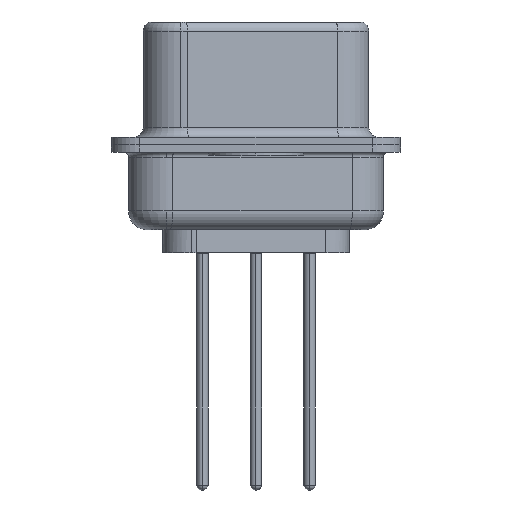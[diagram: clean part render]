
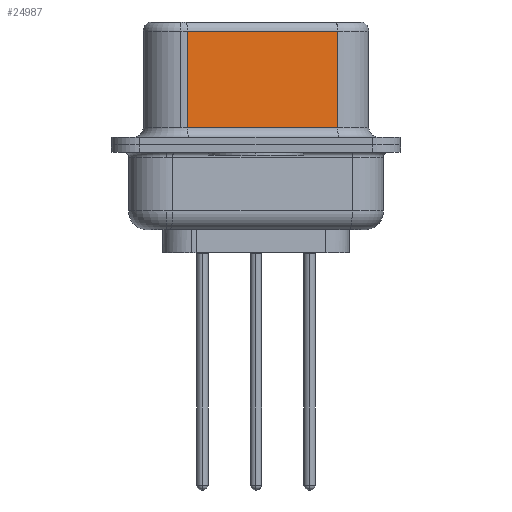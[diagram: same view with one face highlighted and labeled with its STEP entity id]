
A CAD part, left-side view. The second image highlights one B-rep face of the part: STEP entity #24987.
In plain terms, the highlighted planar face has unit normal (-0.985, -0.174, 0).
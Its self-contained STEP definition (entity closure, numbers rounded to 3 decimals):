
#434 = CARTESIAN_POINT ( 'NONE',  ( 5.132, -4.322, 0.9 ) ) ;
#1413 = ORIENTED_EDGE ( 'NONE', *, *, #6745, .T. ) ;
#2491 = VECTOR ( 'NONE', #8895, 1000. ) ;
#4350 = EDGE_CURVE ( 'NONE', #9837, #22912, #19893, .T. ) ;
#5107 = DIRECTION ( 'NONE',  ( 0., 0., -1. ) ) ;
#5774 = DIRECTION ( 'NONE',  ( 0.985, 0.174, 0. ) ) ;
#5904 = CARTESIAN_POINT ( 'NONE',  ( 5.132, -4.322, 6.52 ) ) ;
#6505 = VERTEX_POINT ( 'NONE', #16084 ) ;
#6745 = EDGE_CURVE ( 'NONE', #22912, #12935, #11440, .T. ) ;
#8169 = EDGE_CURVE ( 'NONE', #12935, #6505, #19488, .T. ) ;
#8642 = CARTESIAN_POINT ( 'NONE',  ( 3.73, 3.628, 0.9 ) ) ;
#8895 = DIRECTION ( 'NONE',  ( 0.174, -0.985, 0. ) ) ;
#9201 = CARTESIAN_POINT ( 'NONE',  ( 3.73, 3.628, 6.52 ) ) ;
#9265 = EDGE_LOOP ( 'NONE', ( #17857, #27466, #1413, #10239 ) ) ;
#9506 = VECTOR ( 'NONE', #10115, 1000. ) ;
#9744 = VECTOR ( 'NONE', #20174, 1000. ) ;
#9837 = VERTEX_POINT ( 'NONE', #12917 ) ;
#10115 = DIRECTION ( 'NONE',  ( -0.174, 0.985, 0. ) ) ;
#10239 = ORIENTED_EDGE ( 'NONE', *, *, #8169, .T. ) ;
#10351 = FACE_OUTER_BOUND ( 'NONE', #9265, .T. ) ;
#11440 = LINE ( 'NONE', #9201, #9744 ) ;
#12150 = EDGE_CURVE ( 'NONE', #9837, #6505, #26519, .T. ) ;
#12917 = CARTESIAN_POINT ( 'NONE',  ( 5.132, -4.322, 6.02 ) ) ;
#12935 = VERTEX_POINT ( 'NONE', #8642 ) ;
#14280 = DIRECTION ( 'NONE',  ( -0.174, 0.985, 0. ) ) ;
#14830 = PLANE ( 'NONE',  #27312 ) ;
#16084 = CARTESIAN_POINT ( 'NONE',  ( 5.132, -4.322, 0.9 ) ) ;
#16190 = VECTOR ( 'NONE', #5107, 1000. ) ;
#17857 = ORIENTED_EDGE ( 'NONE', *, *, #12150, .F. ) ;
#19488 = LINE ( 'NONE', #434, #2491 ) ;
#19893 = LINE ( 'NONE', #26282, #9506 ) ;
#20174 = DIRECTION ( 'NONE',  ( 0., 0., -1. ) ) ;
#22912 = VERTEX_POINT ( 'NONE', #27190 ) ;
#24987 = ADVANCED_FACE ( 'NONE', ( #10351 ), #14830, .F. ) ;
#26248 = CARTESIAN_POINT ( 'NONE',  ( 5.132, -4.322, 6.52 ) ) ;
#26282 = CARTESIAN_POINT ( 'NONE',  ( 5.132, -4.322, 6.02 ) ) ;
#26519 = LINE ( 'NONE', #26248, #16190 ) ;
#27190 = CARTESIAN_POINT ( 'NONE',  ( 3.73, 3.628, 6.02 ) ) ;
#27312 = AXIS2_PLACEMENT_3D ( 'NONE', #5904, #5774, #14280 ) ;
#27466 = ORIENTED_EDGE ( 'NONE', *, *, #4350, .T. ) ;
